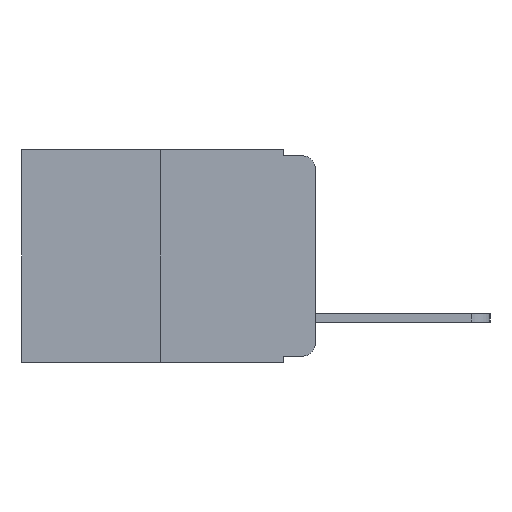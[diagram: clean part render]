
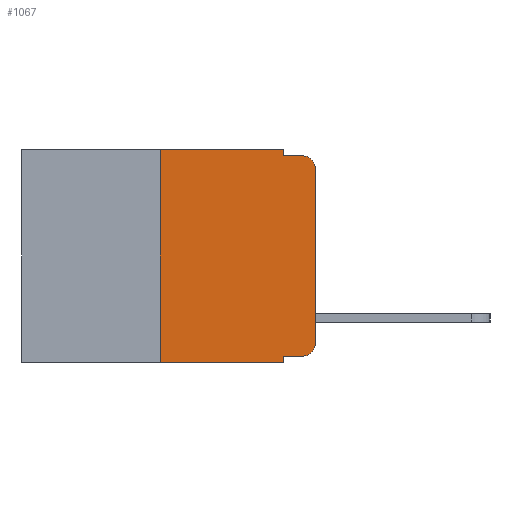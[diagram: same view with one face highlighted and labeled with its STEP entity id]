
A CAD part, left-side view. The second image highlights one B-rep face of the part: STEP entity #1067.
In plain terms, the highlighted planar face has unit normal (-1, 0, 0).
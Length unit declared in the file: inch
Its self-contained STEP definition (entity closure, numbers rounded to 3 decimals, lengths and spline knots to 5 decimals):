
#63 = VERTEX_POINT ( 'NONE', #3522 ) ;
#204 = LINE ( 'NONE', #9032, #2934 ) ;
#457 = CARTESIAN_POINT ( 'NONE',  ( 0., 0.051, -0.333 ) ) ;
#488 = VERTEX_POINT ( 'NONE', #457 ) ;
#524 = LINE ( 'NONE', #6642, #7369 ) ;
#538 = VECTOR ( 'NONE', #1732, 39.37008 ) ;
#563 = ORIENTED_EDGE ( 'NONE', *, *, #5367, .T. ) ;
#594 = ORIENTED_EDGE ( 'NONE', *, *, #4829, .T. ) ;
#638 = ORIENTED_EDGE ( 'NONE', *, *, #5002, .F. ) ;
#653 = ORIENTED_EDGE ( 'NONE', *, *, #5402, .F. ) ;
#686 = ORIENTED_EDGE ( 'NONE', *, *, #11233, .F. ) ;
#785 = ORIENTED_EDGE ( 'NONE', *, *, #4808, .F. ) ;
#878 = CARTESIAN_POINT ( 'NONE',  ( 0., 0.051, 0. ) ) ;
#897 = ORIENTED_EDGE ( 'NONE', *, *, #3650, .T. ) ;
#1045 = ORIENTED_EDGE ( 'NONE', *, *, #5479, .F. ) ;
#1067 = ADVANCED_FACE ( 'NONE', ( #1728 ), #9628, .F. ) ;
#1109 = DIRECTION ( 'NONE',  ( 0., 0., -1. ) ) ;
#1728 = FACE_OUTER_BOUND ( 'NONE', #3841, .T. ) ;
#1732 = DIRECTION ( 'NONE',  ( 0., -1., 0. ) ) ;
#1821 = CARTESIAN_POINT ( 'NONE',  ( 0., 0.051, 0. ) ) ;
#2000 = LINE ( 'NONE', #5383, #2277 ) ;
#2277 = VECTOR ( 'NONE', #8604, 39.37008 ) ;
#2312 = VERTEX_POINT ( 'NONE', #7310 ) ;
#2584 = LINE ( 'NONE', #878, #7096 ) ;
#2600 = CIRCLE ( 'NONE', #9020, 0.02 ) ;
#2726 = DIRECTION ( 'NONE',  ( 0., 0., -1. ) ) ;
#2884 = DIRECTION ( 'NONE',  ( -1., 0., 0. ) ) ;
#2889 = VECTOR ( 'NONE', #3507, 39.37008 ) ;
#2934 = VECTOR ( 'NONE', #8102, 39.37008 ) ;
#3012 = DIRECTION ( 'NONE',  ( 0., 0., -1. ) ) ;
#3486 = CARTESIAN_POINT ( 'NONE',  ( 0., 0.051, -0.01 ) ) ;
#3507 = DIRECTION ( 'NONE',  ( 0., -1., 0. ) ) ;
#3522 = CARTESIAN_POINT ( 'NONE',  ( 0., 0.25, -0.343 ) ) ;
#3650 = EDGE_CURVE ( 'NONE', #63, #4609, #5596, .T. ) ;
#3753 = VECTOR ( 'NONE', #6718, 39.37008 ) ;
#3841 = EDGE_LOOP ( 'NONE', ( #563, #594, #638, #653, #686, #785, #897, #1045, #7611, #8137 ) ) ;
#3975 = VERTEX_POINT ( 'NONE', #11127 ) ;
#4039 = LINE ( 'NONE', #11083, #3753 ) ;
#4407 = VERTEX_POINT ( 'NONE', #1821 ) ;
#4569 = CARTESIAN_POINT ( 'NONE',  ( 0., 0., -0.03 ) ) ;
#4587 = CARTESIAN_POINT ( 'NONE',  ( 0., 0.02, -0.313 ) ) ;
#4609 = VERTEX_POINT ( 'NONE', #10771 ) ;
#4768 = AXIS2_PLACEMENT_3D ( 'NONE', #4587, #2884, #1109 ) ;
#4808 = EDGE_CURVE ( 'NONE', #63, #3975, #524, .T. ) ;
#4829 = EDGE_CURVE ( 'NONE', #6785, #2312, #2600, .T. ) ;
#4912 = CARTESIAN_POINT ( 'NONE',  ( 0., 0.473, -0.343 ) ) ;
#4960 = VERTEX_POINT ( 'NONE', #6974 ) ;
#5002 = EDGE_CURVE ( 'NONE', #6731, #2312, #2000, .T. ) ;
#5284 = LINE ( 'NONE', #5815, #2889 ) ;
#5367 = EDGE_CURVE ( 'NONE', #5446, #6785, #10385, .T. ) ;
#5383 = CARTESIAN_POINT ( 'NONE',  ( 0., 0.051, -0.01 ) ) ;
#5402 = EDGE_CURVE ( 'NONE', #4407, #6731, #4039, .T. ) ;
#5416 = DIRECTION ( 'NONE',  ( -1., 0., 0. ) ) ;
#5429 = CARTESIAN_POINT ( 'NONE',  ( 0., 0., 0. ) ) ;
#5438 = EDGE_CURVE ( 'NONE', #488, #4960, #5284, .T. ) ;
#5446 = VERTEX_POINT ( 'NONE', #6153 ) ;
#5479 = EDGE_CURVE ( 'NONE', #488, #4609, #2584, .T. ) ;
#5544 = EDGE_CURVE ( 'NONE', #4960, #5446, #10720, .T. ) ;
#5596 = LINE ( 'NONE', #4912, #538 ) ;
#5815 = CARTESIAN_POINT ( 'NONE',  ( 0., 0.051, -0.333 ) ) ;
#6127 = DIRECTION ( 'NONE',  ( 0., 0., -1. ) ) ;
#6153 = CARTESIAN_POINT ( 'NONE',  ( 0., 0., -0.313 ) ) ;
#6642 = CARTESIAN_POINT ( 'NONE',  ( 0., 0.25, 0. ) ) ;
#6654 = DIRECTION ( 'NONE',  ( 0., 0., 1. ) ) ;
#6718 = DIRECTION ( 'NONE',  ( 0., 0., -1. ) ) ;
#6731 = VERTEX_POINT ( 'NONE', #3486 ) ;
#6785 = VERTEX_POINT ( 'NONE', #4569 ) ;
#6974 = CARTESIAN_POINT ( 'NONE',  ( 0., 0.02, -0.333 ) ) ;
#7096 = VECTOR ( 'NONE', #2726, 39.37008 ) ;
#7310 = CARTESIAN_POINT ( 'NONE',  ( 0., 0.02, -0.01 ) ) ;
#7352 = CARTESIAN_POINT ( 'NONE',  ( 0., 0.02, -0.03 ) ) ;
#7369 = VECTOR ( 'NONE', #6654, 39.37008 ) ;
#7611 = ORIENTED_EDGE ( 'NONE', *, *, #5438, .T. ) ;
#7612 = DIRECTION ( 'NONE',  ( 0., 0., 1. ) ) ;
#8102 = DIRECTION ( 'NONE',  ( 0., -1., 0. ) ) ;
#8137 = ORIENTED_EDGE ( 'NONE', *, *, #5544, .T. ) ;
#8319 = VECTOR ( 'NONE', #7612, 39.37008 ) ;
#8604 = DIRECTION ( 'NONE',  ( 0., -1., 0. ) ) ;
#9020 = AXIS2_PLACEMENT_3D ( 'NONE', #7352, #5416, #3012 ) ;
#9032 = CARTESIAN_POINT ( 'NONE',  ( 0., 0.473, 0. ) ) ;
#9583 = CARTESIAN_POINT ( 'NONE',  ( 0., 0.473, 0. ) ) ;
#9628 = PLANE ( 'NONE',  #10825 ) ;
#10128 = DIRECTION ( 'NONE',  ( 1., 0., 0. ) ) ;
#10385 = LINE ( 'NONE', #5429, #8319 ) ;
#10720 = CIRCLE ( 'NONE', #4768, 0.02 ) ;
#10771 = CARTESIAN_POINT ( 'NONE',  ( 0., 0.051, -0.343 ) ) ;
#10825 = AXIS2_PLACEMENT_3D ( 'NONE', #9583, #10128, #6127 ) ;
#11083 = CARTESIAN_POINT ( 'NONE',  ( 0., 0.051, 0. ) ) ;
#11127 = CARTESIAN_POINT ( 'NONE',  ( 0., 0.25, 0. ) ) ;
#11233 = EDGE_CURVE ( 'NONE', #3975, #4407, #204, .T. ) ;
